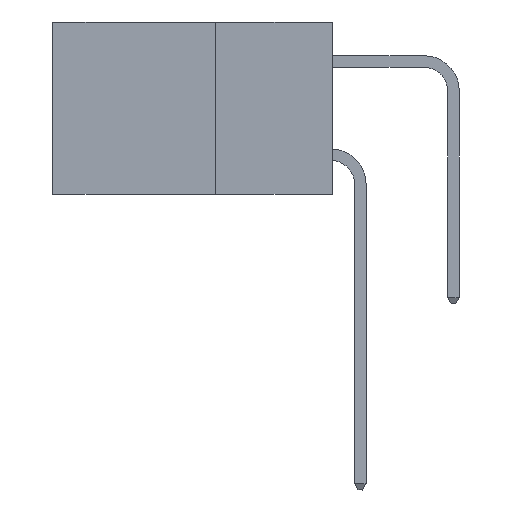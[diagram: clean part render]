
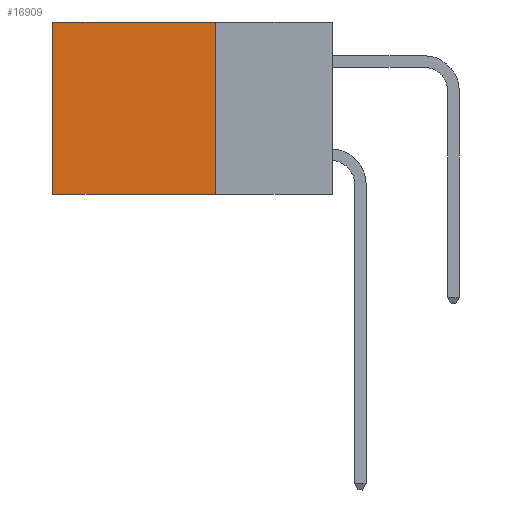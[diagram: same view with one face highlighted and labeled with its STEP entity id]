
A CAD part, left-side view. The second image highlights one B-rep face of the part: STEP entity #16909.
In plain terms, the highlighted planar face has unit normal (-1, 0, 0).
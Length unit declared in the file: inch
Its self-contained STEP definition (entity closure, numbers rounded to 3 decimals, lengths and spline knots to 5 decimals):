
#1162 = VERTEX_POINT ( 'NONE', #9602 ) ;
#2810 = CARTESIAN_POINT ( 'NONE',  ( 0.298, 0.6, 0. ) ) ;
#3298 = VECTOR ( 'NONE', #3576, 39.37008 ) ;
#3576 = DIRECTION ( 'NONE',  ( 0., 0., -1. ) ) ;
#4175 = VECTOR ( 'NONE', #23717, 39.37008 ) ;
#4300 = EDGE_CURVE ( 'NONE', #1162, #23333, #10533, .T. ) ;
#7963 = CARTESIAN_POINT ( 'NONE',  ( 0.298, 0.6, -0.37 ) ) ;
#8380 = VERTEX_POINT ( 'NONE', #7963 ) ;
#9037 = ORIENTED_EDGE ( 'NONE', *, *, #16017, .T. ) ;
#9374 = CARTESIAN_POINT ( 'NONE',  ( 0.298, 0.6, 0. ) ) ;
#9602 = CARTESIAN_POINT ( 'NONE',  ( 0.298, 0.25, 0. ) ) ;
#10251 = DIRECTION ( 'NONE',  ( 1., 0., 0. ) ) ;
#10533 = LINE ( 'NONE', #23541, #4175 ) ;
#11634 = CARTESIAN_POINT ( 'NONE',  ( 0.298, 0.25, 0. ) ) ;
#11961 = DIRECTION ( 'NONE',  ( 0., 1., 0. ) ) ;
#12043 = VECTOR ( 'NONE', #11961, 39.37008 ) ;
#13909 = EDGE_CURVE ( 'NONE', #16336, #8380, #23481, .T. ) ;
#14952 = VECTOR ( 'NONE', #24679, 39.37008 ) ;
#15880 = PLANE ( 'NONE',  #16974 ) ;
#16017 = EDGE_CURVE ( 'NONE', #1162, #16336, #19376, .T. ) ;
#16336 = VERTEX_POINT ( 'NONE', #2810 ) ;
#16466 = LINE ( 'NONE', #23172, #12043 ) ;
#16627 = ORIENTED_EDGE ( 'NONE', *, *, #13909, .T. ) ;
#16909 = ADVANCED_FACE ( 'NONE', ( #24093 ), #15880, .F. ) ;
#16974 = AXIS2_PLACEMENT_3D ( 'NONE', #21501, #10251, #23370 ) ;
#18099 = EDGE_CURVE ( 'NONE', #23333, #8380, #16466, .T. ) ;
#19376 = LINE ( 'NONE', #11634, #14952 ) ;
#19641 = EDGE_LOOP ( 'NONE', ( #16627, #22534, #19782, #9037 ) ) ;
#19782 = ORIENTED_EDGE ( 'NONE', *, *, #4300, .F. ) ;
#21501 = CARTESIAN_POINT ( 'NONE',  ( 0.298, 0.25, 0. ) ) ;
#22534 = ORIENTED_EDGE ( 'NONE', *, *, #18099, .F. ) ;
#23102 = CARTESIAN_POINT ( 'NONE',  ( 0.298, 0.25, -0.37 ) ) ;
#23172 = CARTESIAN_POINT ( 'NONE',  ( 0.298, 0.25, -0.37 ) ) ;
#23333 = VERTEX_POINT ( 'NONE', #23102 ) ;
#23370 = DIRECTION ( 'NONE',  ( 0., 0., -1. ) ) ;
#23481 = LINE ( 'NONE', #9374, #3298 ) ;
#23541 = CARTESIAN_POINT ( 'NONE',  ( 0.298, 0.25, 0. ) ) ;
#23717 = DIRECTION ( 'NONE',  ( 0., 0., -1. ) ) ;
#24093 = FACE_OUTER_BOUND ( 'NONE', #19641, .T. ) ;
#24679 = DIRECTION ( 'NONE',  ( 0., 1., 0. ) ) ;
